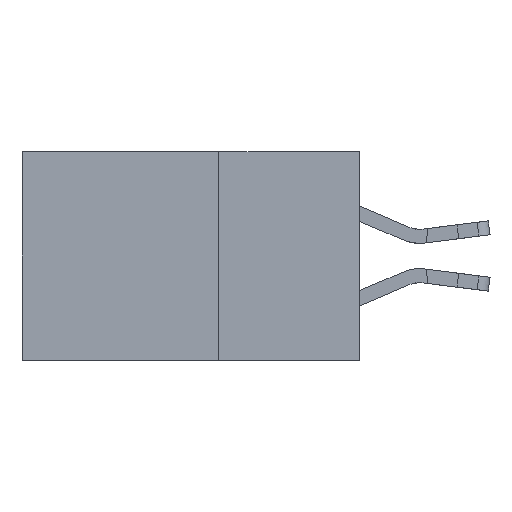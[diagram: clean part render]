
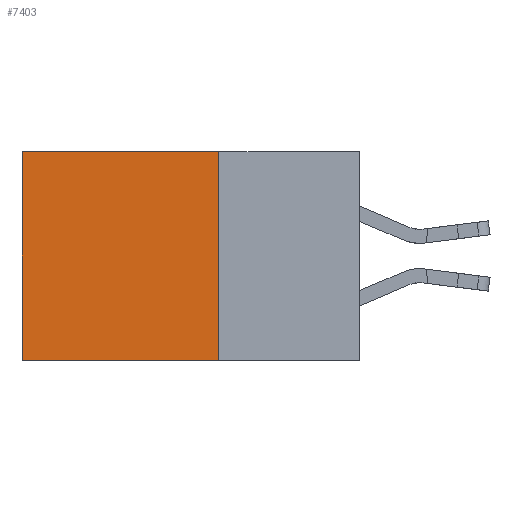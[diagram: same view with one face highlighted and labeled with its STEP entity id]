
A CAD part, left-side view. The second image highlights one B-rep face of the part: STEP entity #7403.
In plain terms, the highlighted planar face has unit normal (-1, 0, 0).
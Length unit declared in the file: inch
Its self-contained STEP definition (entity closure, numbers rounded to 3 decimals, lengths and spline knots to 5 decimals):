
#1222 = EDGE_LOOP ( 'NONE', ( #36696, #17632, #3653, #35571 ) ) ;
#3653 = ORIENTED_EDGE ( 'NONE', *, *, #35073, .F. ) ;
#3878 = LINE ( 'NONE', #35093, #26724 ) ;
#7403 = ADVANCED_FACE ( 'NONE', ( #8065 ), #7588, .F. ) ;
#7496 = LINE ( 'NONE', #10986, #30344 ) ;
#7588 = PLANE ( 'NONE',  #14373 ) ;
#8065 = FACE_OUTER_BOUND ( 'NONE', #1222, .T. ) ;
#10185 = CARTESIAN_POINT ( 'NONE',  ( 0.2875, 0.6, 0. ) ) ;
#10513 = DIRECTION ( 'NONE',  ( 0., 0., -1. ) ) ;
#10986 = CARTESIAN_POINT ( 'NONE',  ( 0.2875, 0.25, -0.37 ) ) ;
#13881 = DIRECTION ( 'NONE',  ( 0., 0., -1. ) ) ;
#13929 = LINE ( 'NONE', #16696, #28217 ) ;
#14373 = AXIS2_PLACEMENT_3D ( 'NONE', #24717, #27600, #10513 ) ;
#16696 = CARTESIAN_POINT ( 'NONE',  ( 0.2875, 0.6, 0. ) ) ;
#17632 = ORIENTED_EDGE ( 'NONE', *, *, #32580, .F. ) ;
#18003 = DIRECTION ( 'NONE',  ( 0., 1., 0. ) ) ;
#19270 = VERTEX_POINT ( 'NONE', #10185 ) ;
#19543 = DIRECTION ( 'NONE',  ( 0., 0., -1. ) ) ;
#20986 = VECTOR ( 'NONE', #13881, 39.37008 ) ;
#21884 = LINE ( 'NONE', #36705, #20986 ) ;
#23410 = EDGE_CURVE ( 'NONE', #19270, #27843, #13929, .T. ) ;
#23497 = CARTESIAN_POINT ( 'NONE',  ( 0.2875, 0.25, 0. ) ) ;
#24717 = CARTESIAN_POINT ( 'NONE',  ( 0.2875, 0.25, 0. ) ) ;
#26724 = VECTOR ( 'NONE', #18003, 39.37008 ) ;
#27600 = DIRECTION ( 'NONE',  ( 1., 0., 0. ) ) ;
#27843 = VERTEX_POINT ( 'NONE', #33889 ) ;
#28089 = DIRECTION ( 'NONE',  ( 0., 1., 0. ) ) ;
#28217 = VECTOR ( 'NONE', #19543, 39.37008 ) ;
#30344 = VECTOR ( 'NONE', #28089, 39.37008 ) ;
#32162 = VERTEX_POINT ( 'NONE', #23497 ) ;
#32580 = EDGE_CURVE ( 'NONE', #35418, #27843, #7496, .T. ) ;
#33889 = CARTESIAN_POINT ( 'NONE',  ( 0.2875, 0.6, -0.37 ) ) ;
#35073 = EDGE_CURVE ( 'NONE', #32162, #35418, #21884, .T. ) ;
#35093 = CARTESIAN_POINT ( 'NONE',  ( 0.2875, 0.25, 0. ) ) ;
#35310 = CARTESIAN_POINT ( 'NONE',  ( 0.2875, 0.25, -0.37 ) ) ;
#35418 = VERTEX_POINT ( 'NONE', #35310 ) ;
#35571 = ORIENTED_EDGE ( 'NONE', *, *, #36703, .T. ) ;
#36696 = ORIENTED_EDGE ( 'NONE', *, *, #23410, .T. ) ;
#36703 = EDGE_CURVE ( 'NONE', #32162, #19270, #3878, .T. ) ;
#36705 = CARTESIAN_POINT ( 'NONE',  ( 0.2875, 0.25, 0. ) ) ;
